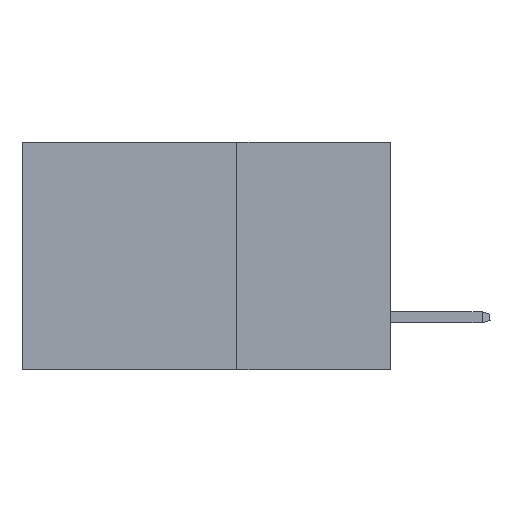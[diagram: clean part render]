
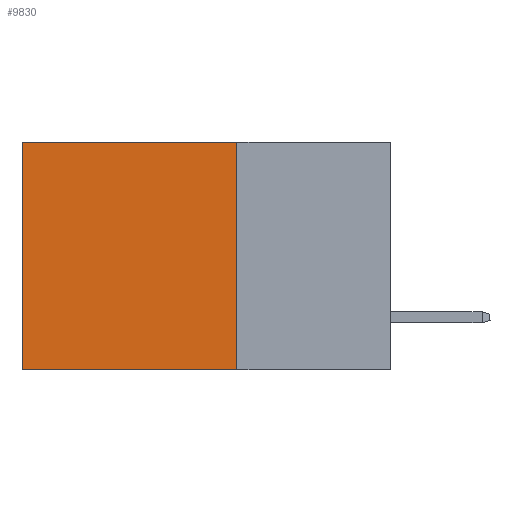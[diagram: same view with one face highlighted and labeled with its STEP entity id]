
A CAD part, left-side view. The second image highlights one B-rep face of the part: STEP entity #9830.
In plain terms, the highlighted planar face has unit normal (-1, 0, 0).
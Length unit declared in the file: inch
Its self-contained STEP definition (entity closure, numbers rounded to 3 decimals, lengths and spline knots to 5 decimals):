
#522 = EDGE_CURVE ( 'NONE', #13184, #2733, #14170, .T. ) ;
#1506 = CARTESIAN_POINT ( 'NONE',  ( 0.2875, 0.25, 0. ) ) ;
#1988 = ORIENTED_EDGE ( 'NONE', *, *, #2705, .T. ) ;
#2036 = LINE ( 'NONE', #1506, #13948 ) ;
#2705 = EDGE_CURVE ( 'NONE', #2733, #15062, #11109, .T. ) ;
#2733 = VERTEX_POINT ( 'NONE', #5339 ) ;
#2937 = ORIENTED_EDGE ( 'NONE', *, *, #11882, .F. ) ;
#3055 = FACE_OUTER_BOUND ( 'NONE', #14990, .T. ) ;
#3577 = AXIS2_PLACEMENT_3D ( 'NONE', #4159, #15479, #5491 ) ;
#3985 = EDGE_CURVE ( 'NONE', #12832, #15062, #11058, .T. ) ;
#4159 = CARTESIAN_POINT ( 'NONE',  ( 0.2875, 0.25, 0. ) ) ;
#5339 = CARTESIAN_POINT ( 'NONE',  ( 0.2875, 0.6, 0. ) ) ;
#5491 = DIRECTION ( 'NONE',  ( 0., 0., -1. ) ) ;
#5551 = PLANE ( 'NONE',  #3577 ) ;
#5788 = ORIENTED_EDGE ( 'NONE', *, *, #522, .T. ) ;
#5934 = CARTESIAN_POINT ( 'NONE',  ( 0.2875, 0.25, 0. ) ) ;
#6181 = DIRECTION ( 'NONE',  ( 0., 1., 0. ) ) ;
#6540 = DIRECTION ( 'NONE',  ( 0., 0., -1. ) ) ;
#7912 = VECTOR ( 'NONE', #14870, 39.37008 ) ;
#8418 = CARTESIAN_POINT ( 'NONE',  ( 0.2875, 0.25, -0.37 ) ) ;
#9751 = VECTOR ( 'NONE', #6540, 39.37008 ) ;
#9830 = ADVANCED_FACE ( 'NONE', ( #3055 ), #5551, .F. ) ;
#10022 = CARTESIAN_POINT ( 'NONE',  ( 0.2875, 0.25, 0. ) ) ;
#10367 = CARTESIAN_POINT ( 'NONE',  ( 0.2875, 0.6, 0. ) ) ;
#10816 = VECTOR ( 'NONE', #6181, 39.37008 ) ;
#11058 = LINE ( 'NONE', #12517, #7912 ) ;
#11109 = LINE ( 'NONE', #10367, #9751 ) ;
#11149 = CARTESIAN_POINT ( 'NONE',  ( 0.2875, 0.6, -0.37 ) ) ;
#11882 = EDGE_CURVE ( 'NONE', #13184, #12832, #2036, .T. ) ;
#12517 = CARTESIAN_POINT ( 'NONE',  ( 0.2875, 0.25, -0.37 ) ) ;
#12832 = VERTEX_POINT ( 'NONE', #8418 ) ;
#13184 = VERTEX_POINT ( 'NONE', #5934 ) ;
#13924 = ORIENTED_EDGE ( 'NONE', *, *, #3985, .F. ) ;
#13948 = VECTOR ( 'NONE', #15312, 39.37008 ) ;
#14170 = LINE ( 'NONE', #10022, #10816 ) ;
#14870 = DIRECTION ( 'NONE',  ( 0., 1., 0. ) ) ;
#14990 = EDGE_LOOP ( 'NONE', ( #1988, #13924, #2937, #5788 ) ) ;
#15062 = VERTEX_POINT ( 'NONE', #11149 ) ;
#15312 = DIRECTION ( 'NONE',  ( 0., 0., -1. ) ) ;
#15479 = DIRECTION ( 'NONE',  ( 1., 0., 0. ) ) ;
